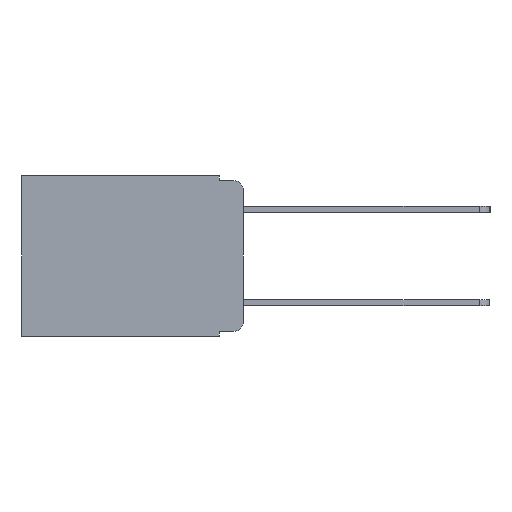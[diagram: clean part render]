
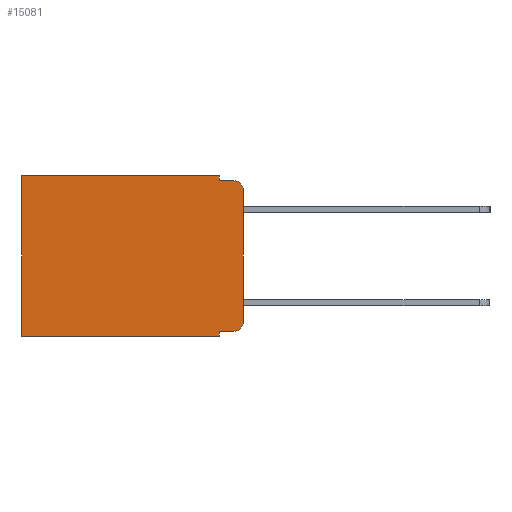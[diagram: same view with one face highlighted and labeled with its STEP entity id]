
A CAD part, left-side view. The second image highlights one B-rep face of the part: STEP entity #15081.
In plain terms, the highlighted planar face has unit normal (-1, 0, 0).
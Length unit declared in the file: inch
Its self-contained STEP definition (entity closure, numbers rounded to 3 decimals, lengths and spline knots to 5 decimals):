
#152 = VERTEX_POINT ( 'NONE', #4731 ) ;
#243 = CARTESIAN_POINT ( 'NONE',  ( 0.298, 0.051, 0. ) ) ;
#300 = DIRECTION ( 'NONE',  ( 0., -1., 0. ) ) ;
#346 = VERTEX_POINT ( 'NONE', #8812 ) ;
#594 = VECTOR ( 'NONE', #13325, 39.37008 ) ;
#817 = DIRECTION ( 'NONE',  ( 0., 0., -1. ) ) ;
#827 = DIRECTION ( 'NONE',  ( 0., 1., 0. ) ) ;
#1032 = CARTESIAN_POINT ( 'NONE',  ( 0.298, 0., 0. ) ) ;
#1850 = CARTESIAN_POINT ( 'NONE',  ( 0.298, 0.051, 0. ) ) ;
#2010 = LINE ( 'NONE', #243, #13983 ) ;
#2308 = DIRECTION ( 'NONE',  ( 0., 0., -1. ) ) ;
#2354 = LINE ( 'NONE', #1850, #11306 ) ;
#2377 = LINE ( 'NONE', #7996, #5190 ) ;
#2770 = CIRCLE ( 'NONE', #10211, 0.02 ) ;
#3363 = VERTEX_POINT ( 'NONE', #10928 ) ;
#3551 = CARTESIAN_POINT ( 'NONE',  ( 0.298, 0.051, -0.01 ) ) ;
#3707 = CARTESIAN_POINT ( 'NONE',  ( 0.298, 0.02, -0.03 ) ) ;
#4097 = AXIS2_PLACEMENT_3D ( 'NONE', #5682, #13619, #6831 ) ;
#4133 = CARTESIAN_POINT ( 'NONE',  ( 0.298, 0., -0.343 ) ) ;
#4272 = ORIENTED_EDGE ( 'NONE', *, *, #9176, .T. ) ;
#4288 = ORIENTED_EDGE ( 'NONE', *, *, #10720, .F. ) ;
#4397 = ORIENTED_EDGE ( 'NONE', *, *, #7655, .F. ) ;
#4400 = FACE_OUTER_BOUND ( 'NONE', #6625, .T. ) ;
#4462 = EDGE_CURVE ( 'NONE', #6340, #10442, #5803, .T. ) ;
#4493 = DIRECTION ( 'NONE',  ( 0., 0., -1. ) ) ;
#4606 = ORIENTED_EDGE ( 'NONE', *, *, #8438, .F. ) ;
#4610 = ORIENTED_EDGE ( 'NONE', *, *, #6840, .T. ) ;
#4666 = ORIENTED_EDGE ( 'NONE', *, *, #14549, .T. ) ;
#4731 = CARTESIAN_POINT ( 'NONE',  ( 0.298, 0.051, 0. ) ) ;
#4797 = ORIENTED_EDGE ( 'NONE', *, *, #10436, .F. ) ;
#4890 = ORIENTED_EDGE ( 'NONE', *, *, #6062, .F. ) ;
#4938 = DIRECTION ( 'NONE',  ( 0., 0., -1. ) ) ;
#5058 = DIRECTION ( 'NONE',  ( 0., -1., 0. ) ) ;
#5172 = ORIENTED_EDGE ( 'NONE', *, *, #5282, .T. ) ;
#5176 = ORIENTED_EDGE ( 'NONE', *, *, #4462, .T. ) ;
#5190 = VECTOR ( 'NONE', #827, 39.37008 ) ;
#5282 = EDGE_CURVE ( 'NONE', #10798, #6340, #12172, .T. ) ;
#5524 = AXIS2_PLACEMENT_3D ( 'NONE', #9157, #11437, #4493 ) ;
#5682 = CARTESIAN_POINT ( 'NONE',  ( 0.298, 0.02, -0.313 ) ) ;
#5803 = CIRCLE ( 'NONE', #4097, 0.02 ) ;
#5925 = CARTESIAN_POINT ( 'NONE',  ( 0.298, 0.051, -0.333 ) ) ;
#6062 = EDGE_CURVE ( 'NONE', #10798, #3363, #2354, .T. ) ;
#6340 = VERTEX_POINT ( 'NONE', #10667 ) ;
#6625 = EDGE_LOOP ( 'NONE', ( #4288, #4272, #4606, #4397, #4666, #4610, #4797, #4890, #5172, #5176 ) ) ;
#6831 = DIRECTION ( 'NONE',  ( 0., 0., -1. ) ) ;
#6840 = EDGE_CURVE ( 'NONE', #10240, #10557, #8975, .T. ) ;
#7366 = CARTESIAN_POINT ( 'NONE',  ( 0.298, 0.473, 0. ) ) ;
#7540 = CARTESIAN_POINT ( 'NONE',  ( 0.298, 0.051, -0.333 ) ) ;
#7655 = EDGE_CURVE ( 'NONE', #152, #12863, #2010, .T. ) ;
#7737 = CARTESIAN_POINT ( 'NONE',  ( 0.298, 0., -0.313 ) ) ;
#7985 = PLANE ( 'NONE',  #5524 ) ;
#7996 = CARTESIAN_POINT ( 'NONE',  ( 0.298, 0., 0. ) ) ;
#8438 = EDGE_CURVE ( 'NONE', #12863, #346, #9221, .T. ) ;
#8812 = CARTESIAN_POINT ( 'NONE',  ( 0.298, 0.02, -0.01 ) ) ;
#8974 = DIRECTION ( 'NONE',  ( 0., 0., -1. ) ) ;
#8975 = LINE ( 'NONE', #14757, #14592 ) ;
#9157 = CARTESIAN_POINT ( 'NONE',  ( 0.298, 0., 0. ) ) ;
#9176 = EDGE_CURVE ( 'NONE', #13357, #346, #2770, .T. ) ;
#9196 = VECTOR ( 'NONE', #300, 39.37008 ) ;
#9221 = LINE ( 'NONE', #10830, #14848 ) ;
#10104 = LINE ( 'NONE', #4133, #594 ) ;
#10211 = AXIS2_PLACEMENT_3D ( 'NONE', #3707, #11814, #4938 ) ;
#10226 = CARTESIAN_POINT ( 'NONE',  ( 0.298, 0.473, -0.343 ) ) ;
#10240 = VERTEX_POINT ( 'NONE', #7366 ) ;
#10436 = EDGE_CURVE ( 'NONE', #3363, #10557, #10104, .T. ) ;
#10442 = VERTEX_POINT ( 'NONE', #7737 ) ;
#10557 = VERTEX_POINT ( 'NONE', #10226 ) ;
#10667 = CARTESIAN_POINT ( 'NONE',  ( 0.298, 0.02, -0.333 ) ) ;
#10720 = EDGE_CURVE ( 'NONE', #13357, #10442, #15175, .T. ) ;
#10798 = VERTEX_POINT ( 'NONE', #5925 ) ;
#10830 = CARTESIAN_POINT ( 'NONE',  ( 0.298, 0.051, -0.01 ) ) ;
#10928 = CARTESIAN_POINT ( 'NONE',  ( 0.298, 0.051, -0.343 ) ) ;
#10940 = DIRECTION ( 'NONE',  ( 0., 0., -1. ) ) ;
#11306 = VECTOR ( 'NONE', #8974, 39.37008 ) ;
#11437 = DIRECTION ( 'NONE',  ( 1., 0., 0. ) ) ;
#11727 = CARTESIAN_POINT ( 'NONE',  ( 0.298, 0., -0.03 ) ) ;
#11814 = DIRECTION ( 'NONE',  ( -1., 0., 0. ) ) ;
#12153 = VECTOR ( 'NONE', #2308, 39.37008 ) ;
#12172 = LINE ( 'NONE', #7540, #9196 ) ;
#12863 = VERTEX_POINT ( 'NONE', #3551 ) ;
#13325 = DIRECTION ( 'NONE',  ( 0., 1., 0. ) ) ;
#13357 = VERTEX_POINT ( 'NONE', #11727 ) ;
#13619 = DIRECTION ( 'NONE',  ( -1., 0., 0. ) ) ;
#13983 = VECTOR ( 'NONE', #10940, 39.37008 ) ;
#14549 = EDGE_CURVE ( 'NONE', #152, #10240, #2377, .T. ) ;
#14592 = VECTOR ( 'NONE', #817, 39.37008 ) ;
#14757 = CARTESIAN_POINT ( 'NONE',  ( 0.298, 0.473, 0. ) ) ;
#14848 = VECTOR ( 'NONE', #5058, 39.37008 ) ;
#15081 = ADVANCED_FACE ( 'NONE', ( #4400 ), #7985, .F. ) ;
#15175 = LINE ( 'NONE', #1032, #12153 ) ;
